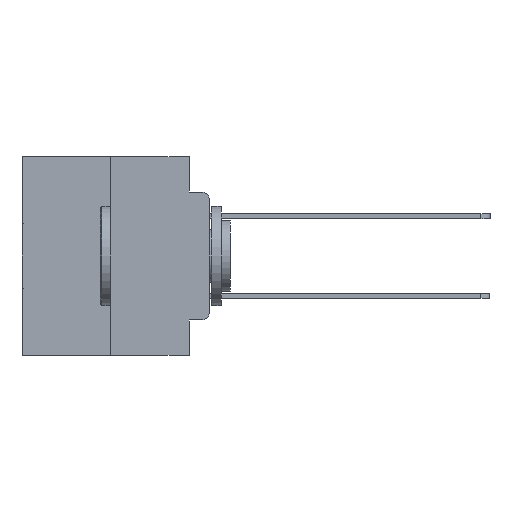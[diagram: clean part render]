
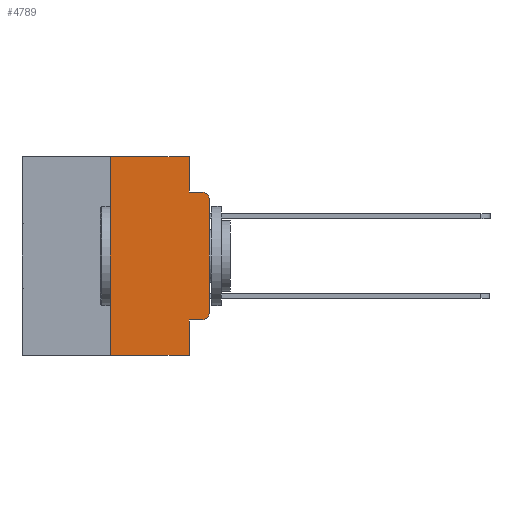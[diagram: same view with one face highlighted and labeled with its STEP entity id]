
A CAD part, left-side view. The second image highlights one B-rep face of the part: STEP entity #4789.
In plain terms, the highlighted planar face has unit normal (-1, 0, 0).
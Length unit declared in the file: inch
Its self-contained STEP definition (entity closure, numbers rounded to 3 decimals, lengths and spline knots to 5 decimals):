
#207 = AXIS2_PLACEMENT_3D ( 'NONE', #7503, #24738, #9999 ) ;
#349 = CARTESIAN_POINT ( 'NONE',  ( 0., 0.051, -0.4115 ) ) ;
#513 = EDGE_CURVE ( 'NONE', #2234, #20622, #19223, .T. ) ;
#712 = VERTEX_POINT ( 'NONE', #21384 ) ;
#760 = VECTOR ( 'NONE', #16526, 39.37008 ) ;
#1500 = DIRECTION ( 'NONE',  ( 0., 0., -1. ) ) ;
#2234 = VERTEX_POINT ( 'NONE', #349 ) ;
#2282 = CIRCLE ( 'NONE', #207, 0.02 ) ;
#2963 = ORIENTED_EDGE ( 'NONE', *, *, #26278, .T. ) ;
#3229 = ORIENTED_EDGE ( 'NONE', *, *, #9143, .F. ) ;
#3717 = CIRCLE ( 'NONE', #9367, 0.02 ) ;
#4054 = EDGE_CURVE ( 'NONE', #2234, #20948, #14938, .T. ) ;
#4162 = DIRECTION ( 'NONE',  ( 0., -1., 0. ) ) ;
#4406 = ORIENTED_EDGE ( 'NONE', *, *, #17461, .F. ) ;
#4442 = CARTESIAN_POINT ( 'NONE',  ( 0., 0.25, 0. ) ) ;
#4789 = ADVANCED_FACE ( 'NONE', ( #26827 ), #20095, .F. ) ;
#5448 = VERTEX_POINT ( 'NONE', #22536 ) ;
#6248 = DIRECTION ( 'NONE',  ( 0., -1., 0. ) ) ;
#6480 = VECTOR ( 'NONE', #25776, 39.37008 ) ;
#6508 = DIRECTION ( 'NONE',  ( 0., 0., -1. ) ) ;
#6650 = CARTESIAN_POINT ( 'NONE',  ( 0., 0.051, -0.0885 ) ) ;
#6772 = DIRECTION ( 'NONE',  ( 0., 0., -1. ) ) ;
#6921 = VERTEX_POINT ( 'NONE', #11120 ) ;
#6947 = ORIENTED_EDGE ( 'NONE', *, *, #20730, .T. ) ;
#7010 = CARTESIAN_POINT ( 'NONE',  ( 0., 0.051, 0. ) ) ;
#7244 = VECTOR ( 'NONE', #6248, 39.37008 ) ;
#7503 = CARTESIAN_POINT ( 'NONE',  ( 0., 0.02, -0.1085 ) ) ;
#7684 = LINE ( 'NONE', #21479, #760 ) ;
#8064 = ORIENTED_EDGE ( 'NONE', *, *, #18508, .F. ) ;
#8950 = DIRECTION ( 'NONE',  ( 0., -1., 0. ) ) ;
#9143 = EDGE_CURVE ( 'NONE', #13417, #19366, #7684, .T. ) ;
#9367 = AXIS2_PLACEMENT_3D ( 'NONE', #31282, #16603, #1500 ) ;
#9961 = ORIENTED_EDGE ( 'NONE', *, *, #14137, .F. ) ;
#9999 = DIRECTION ( 'NONE',  ( 0., 0., -1. ) ) ;
#10284 = CARTESIAN_POINT ( 'NONE',  ( 0., 0.473, 0. ) ) ;
#11120 = CARTESIAN_POINT ( 'NONE',  ( 0., 0.051, 0. ) ) ;
#11887 = EDGE_LOOP ( 'NONE', ( #21569, #6947, #4406, #9961, #8064, #3229, #14381, #25512, #31599, #2963 ) ) ;
#11928 = AXIS2_PLACEMENT_3D ( 'NONE', #10284, #12769, #29961 ) ;
#12730 = VECTOR ( 'NONE', #4162, 39.37008 ) ;
#12769 = DIRECTION ( 'NONE',  ( 1., 0., 0. ) ) ;
#13069 = LINE ( 'NONE', #13414, #6480 ) ;
#13264 = CARTESIAN_POINT ( 'NONE',  ( 0., 0.02, -0.0885 ) ) ;
#13414 = CARTESIAN_POINT ( 'NONE',  ( 0., 0., 0. ) ) ;
#13417 = VERTEX_POINT ( 'NONE', #21144 ) ;
#14137 = EDGE_CURVE ( 'NONE', #6921, #15030, #15250, .T. ) ;
#14381 = ORIENTED_EDGE ( 'NONE', *, *, #30397, .T. ) ;
#14938 = LINE ( 'NONE', #7010, #27268 ) ;
#15030 = VERTEX_POINT ( 'NONE', #29958 ) ;
#15250 = LINE ( 'NONE', #21321, #22560 ) ;
#15702 = CARTESIAN_POINT ( 'NONE',  ( 0., 0.051, -0.5 ) ) ;
#16526 = DIRECTION ( 'NONE',  ( 0., 0., 1. ) ) ;
#16603 = DIRECTION ( 'NONE',  ( -1., 0., 0. ) ) ;
#17205 = VERTEX_POINT ( 'NONE', #13264 ) ;
#17461 = EDGE_CURVE ( 'NONE', #15030, #17205, #25808, .T. ) ;
#18508 = EDGE_CURVE ( 'NONE', #19366, #6921, #20357, .T. ) ;
#19223 = LINE ( 'NONE', #26059, #24975 ) ;
#19366 = VERTEX_POINT ( 'NONE', #4442 ) ;
#20095 = PLANE ( 'NONE',  #11928 ) ;
#20357 = LINE ( 'NONE', #21059, #7244 ) ;
#20622 = VERTEX_POINT ( 'NONE', #21873 ) ;
#20730 = EDGE_CURVE ( 'NONE', #712, #17205, #2282, .T. ) ;
#20948 = VERTEX_POINT ( 'NONE', #15702 ) ;
#21059 = CARTESIAN_POINT ( 'NONE',  ( 0., 0.473, 0. ) ) ;
#21144 = CARTESIAN_POINT ( 'NONE',  ( 0., 0.25, -0.5 ) ) ;
#21321 = CARTESIAN_POINT ( 'NONE',  ( 0., 0.051, 0. ) ) ;
#21384 = CARTESIAN_POINT ( 'NONE',  ( 0., 0., -0.1085 ) ) ;
#21479 = CARTESIAN_POINT ( 'NONE',  ( 0., 0.25, 0. ) ) ;
#21569 = ORIENTED_EDGE ( 'NONE', *, *, #27343, .T. ) ;
#21873 = CARTESIAN_POINT ( 'NONE',  ( 0., 0.02, -0.4115 ) ) ;
#22536 = CARTESIAN_POINT ( 'NONE',  ( 0., 0., -0.3915 ) ) ;
#22560 = VECTOR ( 'NONE', #6508, 39.37008 ) ;
#24738 = DIRECTION ( 'NONE',  ( -1., 0., 0. ) ) ;
#24975 = VECTOR ( 'NONE', #25028, 39.37008 ) ;
#25028 = DIRECTION ( 'NONE',  ( 0., -1., 0. ) ) ;
#25185 = VECTOR ( 'NONE', #8950, 39.37008 ) ;
#25512 = ORIENTED_EDGE ( 'NONE', *, *, #4054, .F. ) ;
#25776 = DIRECTION ( 'NONE',  ( 0., 0., 1. ) ) ;
#25808 = LINE ( 'NONE', #6650, #12730 ) ;
#26059 = CARTESIAN_POINT ( 'NONE',  ( 0., 0.051, -0.4115 ) ) ;
#26278 = EDGE_CURVE ( 'NONE', #20622, #5448, #3717, .T. ) ;
#26827 = FACE_OUTER_BOUND ( 'NONE', #11887, .T. ) ;
#27268 = VECTOR ( 'NONE', #6772, 39.37008 ) ;
#27343 = EDGE_CURVE ( 'NONE', #5448, #712, #13069, .T. ) ;
#29958 = CARTESIAN_POINT ( 'NONE',  ( 0., 0.051, -0.0885 ) ) ;
#29961 = DIRECTION ( 'NONE',  ( 0., 0., -1. ) ) ;
#30397 = EDGE_CURVE ( 'NONE', #13417, #20948, #31695, .T. ) ;
#31009 = CARTESIAN_POINT ( 'NONE',  ( 0., 0.473, -0.5 ) ) ;
#31282 = CARTESIAN_POINT ( 'NONE',  ( 0., 0.02, -0.3915 ) ) ;
#31599 = ORIENTED_EDGE ( 'NONE', *, *, #513, .T. ) ;
#31695 = LINE ( 'NONE', #31009, #25185 ) ;
